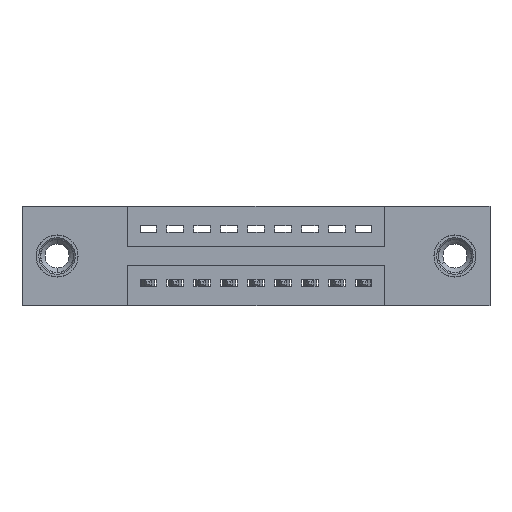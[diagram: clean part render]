
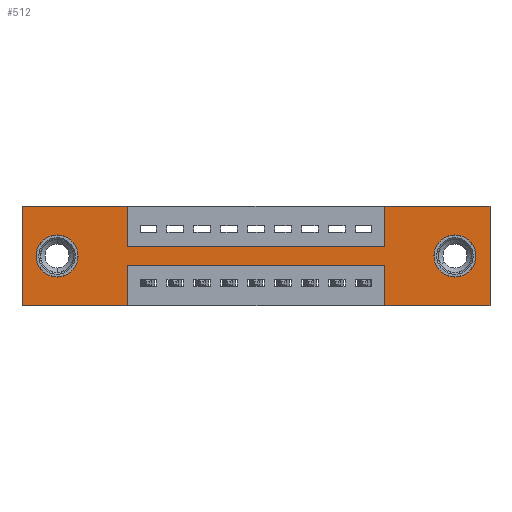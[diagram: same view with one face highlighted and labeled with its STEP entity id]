
A CAD part, front view. The second image highlights one B-rep face of the part: STEP entity #512.
In plain terms, the highlighted planar face has unit normal (0, -1, 0).
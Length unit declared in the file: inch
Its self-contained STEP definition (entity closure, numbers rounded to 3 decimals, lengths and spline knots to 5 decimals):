
#8 = VERTEX_POINT ( 'NONE', #11967 ) ;
#29 = CARTESIAN_POINT ( 'NONE',  ( 0., 0., 0. ) ) ;
#84 = ORIENTED_EDGE ( 'NONE', *, *, #1515, .F. ) ;
#286 = ORIENTED_EDGE ( 'NONE', *, *, #7061, .F. ) ;
#408 = AXIS2_PLACEMENT_3D ( 'NONE', #858, #12350, #2894 ) ;
#512 = ADVANCED_FACE ( 'NONE', ( #10004, #9549, #5658 ), #7059, .T. ) ;
#540 = AXIS2_PLACEMENT_3D ( 'NONE', #2332, #10922, #1492 ) ;
#634 = CIRCLE ( 'NONE', #540, 0.078 ) ;
#636 = CARTESIAN_POINT ( 'NONE',  ( 0.3925, 0., -0.22 ) ) ;
#748 = ORIENTED_EDGE ( 'NONE', *, *, #9023, .F. ) ;
#858 = CARTESIAN_POINT ( 'NONE',  ( 0.13, 0., -0.185 ) ) ;
#959 = CARTESIAN_POINT ( 'NONE',  ( 1.605, 0., -0.263 ) ) ;
#1051 = EDGE_CURVE ( 'NONE', #11370, #6279, #11791, .T. ) ;
#1152 = DIRECTION ( 'NONE',  ( 1., 0., 0. ) ) ;
#1375 = VECTOR ( 'NONE', #9311, 39.37008 ) ;
#1478 = DIRECTION ( 'NONE',  ( 0., 0., 1. ) ) ;
#1492 = DIRECTION ( 'NONE',  ( 0., 0., 1. ) ) ;
#1515 = EDGE_CURVE ( 'NONE', #8567, #6711, #3662, .T. ) ;
#1615 = ORIENTED_EDGE ( 'NONE', *, *, #10927, .F. ) ;
#1702 = VERTEX_POINT ( 'NONE', #8988 ) ;
#1884 = DIRECTION ( 'NONE',  ( -1., 0., 0. ) ) ;
#1944 = VERTEX_POINT ( 'NONE', #2741 ) ;
#2290 = EDGE_CURVE ( 'NONE', #11658, #11370, #2301, .T. ) ;
#2301 = LINE ( 'NONE', #5984, #2598 ) ;
#2332 = CARTESIAN_POINT ( 'NONE',  ( 0.13, 0., -0.185 ) ) ;
#2342 = VERTEX_POINT ( 'NONE', #9229 ) ;
#2358 = CARTESIAN_POINT ( 'NONE',  ( 1.605, 0., -0.185 ) ) ;
#2522 = LINE ( 'NONE', #6331, #9433 ) ;
#2532 = VECTOR ( 'NONE', #5812, 39.37008 ) ;
#2598 = VECTOR ( 'NONE', #10871, 39.37008 ) ;
#2741 = CARTESIAN_POINT ( 'NONE',  ( 0.3925, 0., -0.22 ) ) ;
#2752 = EDGE_CURVE ( 'NONE', #1944, #12116, #7363, .T. ) ;
#2782 = AXIS2_PLACEMENT_3D ( 'NONE', #8334, #3561, #10270 ) ;
#2894 = DIRECTION ( 'NONE',  ( 0., 0., 1. ) ) ;
#2922 = CARTESIAN_POINT ( 'NONE',  ( 1.3425, 0., -0.37 ) ) ;
#2925 = ORIENTED_EDGE ( 'NONE', *, *, #1051, .F. ) ;
#2966 = DIRECTION ( 'NONE',  ( 1., 0., 0. ) ) ;
#2967 = CARTESIAN_POINT ( 'NONE',  ( 0.3925, 0., -0.37 ) ) ;
#2968 = ORIENTED_EDGE ( 'NONE', *, *, #5764, .F. ) ;
#3037 = CARTESIAN_POINT ( 'NONE',  ( 0., 0., -0.37 ) ) ;
#3294 = LINE ( 'NONE', #6592, #2532 ) ;
#3310 = EDGE_CURVE ( 'NONE', #2342, #8, #634, .T. ) ;
#3332 = DIRECTION ( 'NONE',  ( 0., 0., -1. ) ) ;
#3501 = ORIENTED_EDGE ( 'NONE', *, *, #11641, .F. ) ;
#3561 = DIRECTION ( 'NONE',  ( 0., 1., 0. ) ) ;
#3662 = LINE ( 'NONE', #7648, #11013 ) ;
#3956 = CARTESIAN_POINT ( 'NONE',  ( 0.3925, 0., -0.15 ) ) ;
#4068 = VERTEX_POINT ( 'NONE', #3956 ) ;
#4125 = CARTESIAN_POINT ( 'NONE',  ( 1.735, 0., 0. ) ) ;
#4210 = ORIENTED_EDGE ( 'NONE', *, *, #5066, .T. ) ;
#4315 = DIRECTION ( 'NONE',  ( 0., -1., 0. ) ) ;
#4442 = DIRECTION ( 'NONE',  ( 0., 0., -1. ) ) ;
#4570 = CARTESIAN_POINT ( 'NONE',  ( 1.735, 0., 0. ) ) ;
#5063 = VECTOR ( 'NONE', #1884, 39.37008 ) ;
#5066 = EDGE_CURVE ( 'NONE', #8, #2342, #6579, .T. ) ;
#5285 = VECTOR ( 'NONE', #2966, 39.37008 ) ;
#5437 = VECTOR ( 'NONE', #1478, 39.37008 ) ;
#5607 = ORIENTED_EDGE ( 'NONE', *, *, #5931, .F. ) ;
#5658 = FACE_OUTER_BOUND ( 'NONE', #10124, .T. ) ;
#5764 = EDGE_CURVE ( 'NONE', #8883, #7822, #3294, .T. ) ;
#5791 = CARTESIAN_POINT ( 'NONE',  ( 0., 0., -0.37 ) ) ;
#5812 = DIRECTION ( 'NONE',  ( 0., 0., 1. ) ) ;
#5915 = CARTESIAN_POINT ( 'NONE',  ( 1.3425, 0., 0. ) ) ;
#5931 = EDGE_CURVE ( 'NONE', #1702, #4068, #2522, .T. ) ;
#5975 = ORIENTED_EDGE ( 'NONE', *, *, #6805, .F. ) ;
#5984 = CARTESIAN_POINT ( 'NONE',  ( 1.3425, 0., 0. ) ) ;
#6017 = CARTESIAN_POINT ( 'NONE',  ( 1.735, 0., -0.37 ) ) ;
#6083 = VECTOR ( 'NONE', #1152, 39.37008 ) ;
#6121 = CARTESIAN_POINT ( 'NONE',  ( 0.3925, 0., -0.37 ) ) ;
#6184 = LINE ( 'NONE', #7242, #5437 ) ;
#6279 = VERTEX_POINT ( 'NONE', #4125 ) ;
#6331 = CARTESIAN_POINT ( 'NONE',  ( 0.3925, 0., 0. ) ) ;
#6402 = ORIENTED_EDGE ( 'NONE', *, *, #9407, .T. ) ;
#6579 = CIRCLE ( 'NONE', #408, 0.078 ) ;
#6592 = CARTESIAN_POINT ( 'NONE',  ( 0., 0., 0. ) ) ;
#6711 = VERTEX_POINT ( 'NONE', #2922 ) ;
#6805 = EDGE_CURVE ( 'NONE', #12116, #8883, #10905, .T. ) ;
#7059 = PLANE ( 'NONE',  #11926 ) ;
#7061 = EDGE_CURVE ( 'NONE', #4068, #11658, #8057, .T. ) ;
#7163 = DIRECTION ( 'NONE',  ( 0., 1., 0. ) ) ;
#7177 = EDGE_LOOP ( 'NONE', ( #4210, #11473 ) ) ;
#7242 = CARTESIAN_POINT ( 'NONE',  ( 1.3425, 0., -0.37 ) ) ;
#7288 = DIRECTION ( 'NONE',  ( 0., 0., -1. ) ) ;
#7305 = EDGE_LOOP ( 'NONE', ( #6402, #8600 ) ) ;
#7360 = LINE ( 'NONE', #8693, #5285 ) ;
#7363 = LINE ( 'NONE', #6121, #11276 ) ;
#7494 = CIRCLE ( 'NONE', #2782, 0.078 ) ;
#7648 = CARTESIAN_POINT ( 'NONE',  ( 0., 0., -0.37 ) ) ;
#7822 = VERTEX_POINT ( 'NONE', #29 ) ;
#7898 = CARTESIAN_POINT ( 'NONE',  ( 0., 0., 0. ) ) ;
#8042 = DIRECTION ( 'NONE',  ( 1., 0., 0. ) ) ;
#8057 = LINE ( 'NONE', #10016, #12413 ) ;
#8111 = LINE ( 'NONE', #636, #8727 ) ;
#8334 = CARTESIAN_POINT ( 'NONE',  ( 1.605, 0., -0.185 ) ) ;
#8454 = AXIS2_PLACEMENT_3D ( 'NONE', #2358, #7163, #11470 ) ;
#8567 = VERTEX_POINT ( 'NONE', #6017 ) ;
#8600 = ORIENTED_EDGE ( 'NONE', *, *, #11772, .T. ) ;
#8623 = DIRECTION ( 'NONE',  ( -1., 0., 0. ) ) ;
#8693 = CARTESIAN_POINT ( 'NONE',  ( 0., 0., 0. ) ) ;
#8727 = VECTOR ( 'NONE', #10037, 39.37008 ) ;
#8883 = VERTEX_POINT ( 'NONE', #3037 ) ;
#8988 = CARTESIAN_POINT ( 'NONE',  ( 0.3925, 0., 0. ) ) ;
#9023 = EDGE_CURVE ( 'NONE', #7822, #1702, #7360, .T. ) ;
#9203 = CIRCLE ( 'NONE', #8454, 0.078 ) ;
#9229 = CARTESIAN_POINT ( 'NONE',  ( 0.13, 0., -0.263 ) ) ;
#9311 = DIRECTION ( 'NONE',  ( 0., 0., -1. ) ) ;
#9407 = EDGE_CURVE ( 'NONE', #11874, #9886, #9203, .T. ) ;
#9433 = VECTOR ( 'NONE', #4442, 39.37008 ) ;
#9549 = FACE_BOUND ( 'NONE', #7177, .T. ) ;
#9886 = VERTEX_POINT ( 'NONE', #959 ) ;
#9915 = EDGE_CURVE ( 'NONE', #6711, #12361, #6184, .T. ) ;
#10004 = FACE_BOUND ( 'NONE', #7305, .T. ) ;
#10016 = CARTESIAN_POINT ( 'NONE',  ( 0.3925, 0., -0.15 ) ) ;
#10037 = DIRECTION ( 'NONE',  ( -1., 0., 0. ) ) ;
#10072 = CARTESIAN_POINT ( 'NONE',  ( 0., 0., -0.37 ) ) ;
#10124 = EDGE_LOOP ( 'NONE', ( #11482, #3501, #11418, #84, #1615, #2925, #10282, #286, #5607, #748, #2968, #5975 ) ) ;
#10270 = DIRECTION ( 'NONE',  ( 0., 0., -1. ) ) ;
#10282 = ORIENTED_EDGE ( 'NONE', *, *, #2290, .F. ) ;
#10871 = DIRECTION ( 'NONE',  ( 0., 0., 1. ) ) ;
#10905 = LINE ( 'NONE', #5791, #5063 ) ;
#10922 = DIRECTION ( 'NONE',  ( 0., 1., 0. ) ) ;
#10927 = EDGE_CURVE ( 'NONE', #6279, #8567, #10971, .T. ) ;
#10971 = LINE ( 'NONE', #4570, #1375 ) ;
#11013 = VECTOR ( 'NONE', #8623, 39.37008 ) ;
#11276 = VECTOR ( 'NONE', #3332, 39.37008 ) ;
#11370 = VERTEX_POINT ( 'NONE', #5915 ) ;
#11418 = ORIENTED_EDGE ( 'NONE', *, *, #9915, .F. ) ;
#11470 = DIRECTION ( 'NONE',  ( 0., 0., -1. ) ) ;
#11473 = ORIENTED_EDGE ( 'NONE', *, *, #3310, .T. ) ;
#11482 = ORIENTED_EDGE ( 'NONE', *, *, #2752, .F. ) ;
#11641 = EDGE_CURVE ( 'NONE', #12361, #1944, #8111, .T. ) ;
#11651 = CARTESIAN_POINT ( 'NONE',  ( 1.3425, 0., -0.22 ) ) ;
#11658 = VERTEX_POINT ( 'NONE', #12217 ) ;
#11772 = EDGE_CURVE ( 'NONE', #9886, #11874, #7494, .T. ) ;
#11791 = LINE ( 'NONE', #7898, #6083 ) ;
#11874 = VERTEX_POINT ( 'NONE', #12421 ) ;
#11926 = AXIS2_PLACEMENT_3D ( 'NONE', #10072, #4315, #7288 ) ;
#11967 = CARTESIAN_POINT ( 'NONE',  ( 0.13, 0., -0.107 ) ) ;
#12116 = VERTEX_POINT ( 'NONE', #2967 ) ;
#12217 = CARTESIAN_POINT ( 'NONE',  ( 1.3425, 0., -0.15 ) ) ;
#12350 = DIRECTION ( 'NONE',  ( 0., 1., 0. ) ) ;
#12361 = VERTEX_POINT ( 'NONE', #11651 ) ;
#12413 = VECTOR ( 'NONE', #8042, 39.37008 ) ;
#12421 = CARTESIAN_POINT ( 'NONE',  ( 1.605, 0., -0.107 ) ) ;
